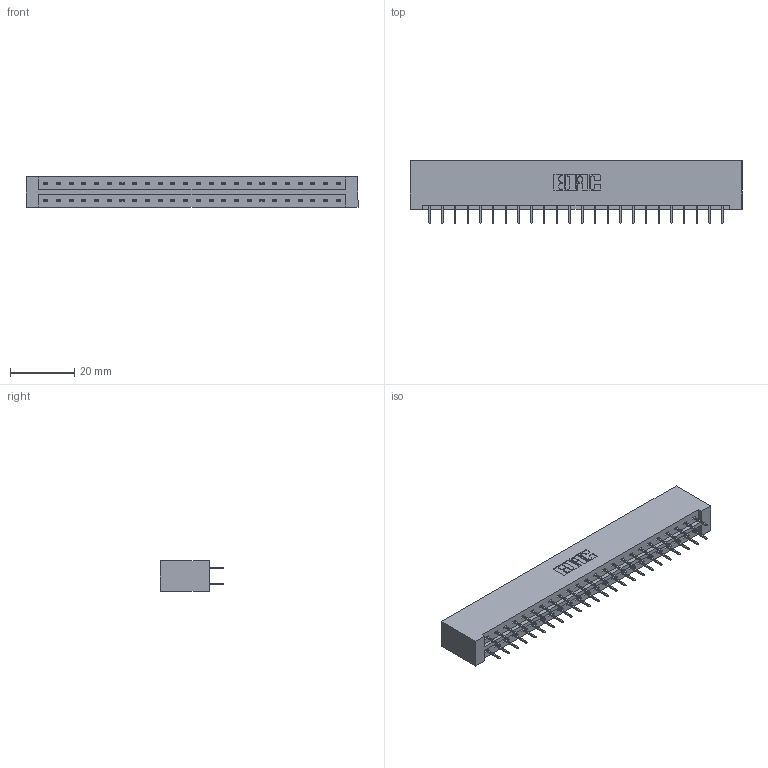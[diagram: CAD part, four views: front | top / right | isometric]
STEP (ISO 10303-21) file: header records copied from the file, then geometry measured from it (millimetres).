
FILE_DESCRIPTION (( 'STEP AP203' ), '1' );
FILE_NAME ('833-048-524-201.STEP', '2020-06-04T15:44:11', ( '' ), ( '' ), 'SwSTEP 2.0', 'SolidWorks 2020', '' );
FILE_SCHEMA (( 'CONFIG_CONTROL_DESIGN' ));
Length unit declared in the file: inch
Products named in the file (3): 833 Part_Lugless; 833-048-524-201; 345-292-001_345-293-124
Assembly tree (49 placements, depth 2):
  833-048-524-201
    833 Part_Lugless
    345-292-001_345-293-124  x48
Bounding box: 103.35 x 19.69 x 9.4 mm (x, y, z)
Volume: 10943 mm3; surface area: 12550.2 mm2
Topology: 49 solids, 49 shells, 2794 faces, 7919 edges, 5086 vertices
Faces by surface type: plane 2082, cylinder 712
Entity records: 17565 total; most frequent: CARTESIAN_POINT 2930, ORIENTED_EDGE 2866, DIRECTION 2529, EDGE_CURVE 1433, LINE 1317, VECTOR 1317, VERTEX_POINT 950, AXIS2_PLACEMENT_3D 606
